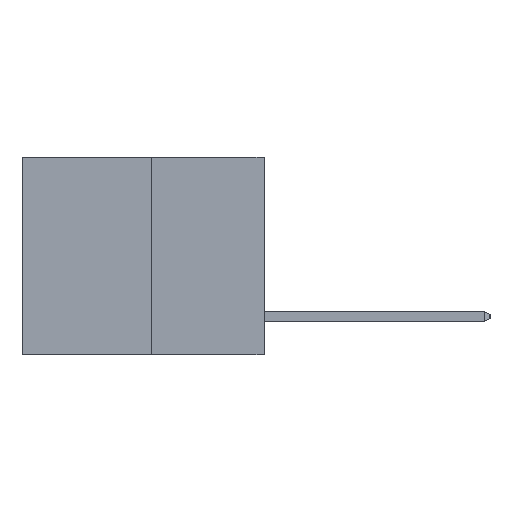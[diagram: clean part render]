
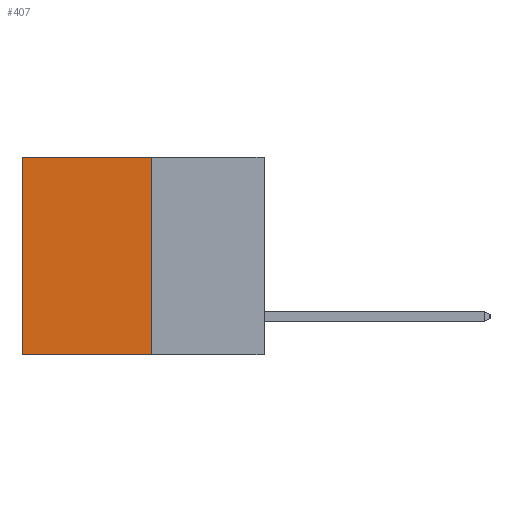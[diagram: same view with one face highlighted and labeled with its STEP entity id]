
A CAD part, left-side view. The second image highlights one B-rep face of the part: STEP entity #407.
In plain terms, the highlighted planar face has unit normal (-1, 0, 0).
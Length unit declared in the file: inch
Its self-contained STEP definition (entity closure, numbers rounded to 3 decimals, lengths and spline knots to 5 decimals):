
#407 = ADVANCED_FACE ( 'NONE', ( #8962 ), #12086, .F. ) ;
#462 = CARTESIAN_POINT ( 'NONE',  ( 0.3165, 0.28, -0.49 ) ) ;
#671 = CARTESIAN_POINT ( 'NONE',  ( 0.3165, 0.28, 0. ) ) ;
#1303 = VERTEX_POINT ( 'NONE', #6372 ) ;
#1715 = EDGE_CURVE ( 'NONE', #11984, #6094, #8903, .T. ) ;
#1719 = EDGE_LOOP ( 'NONE', ( #5838, #4546, #7319, #11794 ) ) ;
#1962 = VECTOR ( 'NONE', #16393, 39.37008 ) ;
#2340 = CARTESIAN_POINT ( 'NONE',  ( 0.3165, 0.28, -0.49 ) ) ;
#2415 = EDGE_CURVE ( 'NONE', #11984, #1303, #7220, .T. ) ;
#4546 = ORIENTED_EDGE ( 'NONE', *, *, #13577, .F. ) ;
#5572 = VECTOR ( 'NONE', #8557, 39.37008 ) ;
#5605 = VECTOR ( 'NONE', #11517, 39.37008 ) ;
#5648 = CARTESIAN_POINT ( 'NONE',  ( 0.3165, 0.28, -0.49 ) ) ;
#5838 = ORIENTED_EDGE ( 'NONE', *, *, #12600, .T. ) ;
#6042 = LINE ( 'NONE', #2340, #5605 ) ;
#6094 = VERTEX_POINT ( 'NONE', #15052 ) ;
#6372 = CARTESIAN_POINT ( 'NONE',  ( 0.3165, 0.6, 0. ) ) ;
#7220 = LINE ( 'NONE', #671, #5572 ) ;
#7319 = ORIENTED_EDGE ( 'NONE', *, *, #1715, .F. ) ;
#7650 = CARTESIAN_POINT ( 'NONE',  ( 0.3165, 0.6, -0.49 ) ) ;
#7768 = CARTESIAN_POINT ( 'NONE',  ( 0.3165, 0.28, 0. ) ) ;
#8557 = DIRECTION ( 'NONE',  ( 0., 1., 0. ) ) ;
#8903 = LINE ( 'NONE', #462, #1962 ) ;
#8962 = FACE_OUTER_BOUND ( 'NONE', #1719, .T. ) ;
#10008 = VERTEX_POINT ( 'NONE', #7650 ) ;
#10645 = DIRECTION ( 'NONE',  ( 0., 0., -1. ) ) ;
#11232 = AXIS2_PLACEMENT_3D ( 'NONE', #5648, #14931, #16146 ) ;
#11517 = DIRECTION ( 'NONE',  ( 0., 1., 0. ) ) ;
#11794 = ORIENTED_EDGE ( 'NONE', *, *, #2415, .T. ) ;
#11984 = VERTEX_POINT ( 'NONE', #7768 ) ;
#12086 = PLANE ( 'NONE',  #11232 ) ;
#12600 = EDGE_CURVE ( 'NONE', #1303, #10008, #15751, .T. ) ;
#13577 = EDGE_CURVE ( 'NONE', #6094, #10008, #6042, .T. ) ;
#14495 = VECTOR ( 'NONE', #10645, 39.37008 ) ;
#14931 = DIRECTION ( 'NONE',  ( 1., 0., 0. ) ) ;
#15052 = CARTESIAN_POINT ( 'NONE',  ( 0.3165, 0.28, -0.49 ) ) ;
#15751 = LINE ( 'NONE', #16072, #14495 ) ;
#16072 = CARTESIAN_POINT ( 'NONE',  ( 0.3165, 0.6, -0.49 ) ) ;
#16146 = DIRECTION ( 'NONE',  ( 0., 0., -1. ) ) ;
#16393 = DIRECTION ( 'NONE',  ( 0., 0., -1. ) ) ;
